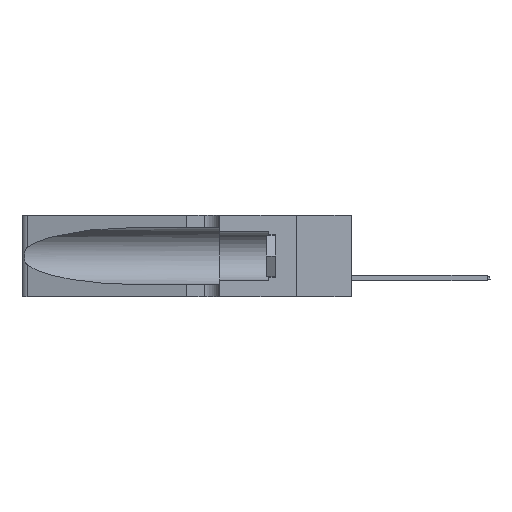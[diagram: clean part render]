
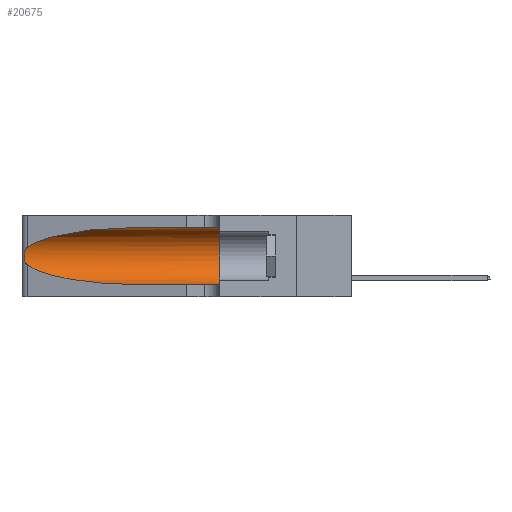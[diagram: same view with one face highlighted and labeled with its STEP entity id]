
A CAD part, left-side view. The second image highlights one B-rep face of the part: STEP entity #20675.
In plain terms, the highlighted cylindrical face has radius 3.308 mm (diameter 6.617 mm), a partial arc.
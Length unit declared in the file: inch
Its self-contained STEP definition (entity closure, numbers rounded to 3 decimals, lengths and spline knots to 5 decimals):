
#195 = ORIENTED_EDGE ( 'NONE', *, *, #631, .F. ) ;
#317 = CARTESIAN_POINT ( 'NONE',  ( 0.1305, 1.61858, 0.05475 ) ) ;
#356 = EDGE_LOOP ( 'NONE', ( #9477, #9032, #9958, #8637, #195, #3630 ) ) ;
#631 = EDGE_CURVE ( 'NONE', #19282, #6868, #21070, .T. ) ;
#970 = CARTESIAN_POINT ( 'NONE',  ( 0.25555, 1.22994, 0.2215 ) ) ;
#1056 = CARTESIAN_POINT ( 'NONE',  ( 0.25639, 1.23184, 0.21858 ) ) ;
#1067 = DIRECTION ( 'NONE',  ( 0., 1., 0. ) ) ;
#1141 = CARTESIAN_POINT ( 'NONE',  ( 0.26075, 1.23896, 0.178 ) ) ;
#1147 = AXIS2_PLACEMENT_3D ( 'NONE', #23636, #1067, #21556 ) ;
#1384 = DIRECTION ( 'NONE',  ( 0., -1., 0. ) ) ;
#1457 =( BOUNDED_CURVE ( )  B_SPLINE_CURVE ( 3, ( #15806, #17543, #21360, #10012 ),
 .UNSPECIFIED., .F., .T. ) 
 B_SPLINE_CURVE_WITH_KNOTS ( ( 4, 4 ),
 ( 3.44316, 4.71239 ),
 .UNSPECIFIED. ) 
 CURVE ( )  GEOMETRIC_REPRESENTATION_ITEM ( )  RATIONAL_B_SPLINE_CURVE ( ( 1., 0.87, 0.87, 1. ) ) 
 REPRESENTATION_ITEM ( '' )  );
#1760 = VECTOR ( 'NONE', #9818, 39.37008 ) ;
#2937 = AXIS2_PLACEMENT_3D ( 'NONE', #8709, #1384, #10711 ) ;
#2951 = CARTESIAN_POINT ( 'NONE',  ( 0.25856, 1.23593, 0.16098 ) ) ;
#3630 = ORIENTED_EDGE ( 'NONE', *, *, #8228, .F. ) ;
#4922 = VERTEX_POINT ( 'NONE', #11655 ) ;
#5606 = EDGE_CURVE ( 'NONE', #18583, #5831, #23296, .T. ) ;
#5831 = VERTEX_POINT ( 'NONE', #16990 ) ;
#6119 = VERTEX_POINT ( 'NONE', #12368 ) ;
#6274 = CARTESIAN_POINT ( 'NONE',  ( 0.18966, 0.96281, 0.31525 ) ) ;
#6665 = CARTESIAN_POINT ( 'NONE',  ( 0.26018, 1.23835, 0.19895 ) ) ;
#6868 = VERTEX_POINT ( 'NONE', #11860 ) ;
#7037 = DIRECTION ( 'NONE',  ( 0., -1., 0. ) ) ;
#7185 = CARTESIAN_POINT ( 'NONE',  ( 0.1305, 1.61858, 0.31525 ) ) ;
#7886 = FACE_OUTER_BOUND ( 'NONE', #356, .T. ) ;
#8228 = EDGE_CURVE ( 'NONE', #6119, #19282, #20398, .T. ) ;
#8541 = CARTESIAN_POINT ( 'NONE',  ( 0.26017, 1.23833, 0.17102 ) ) ;
#8637 = ORIENTED_EDGE ( 'NONE', *, *, #11089, .T. ) ;
#8709 = CARTESIAN_POINT ( 'NONE',  ( 0.1305, 1.61858, 0.185 ) ) ;
#9032 = ORIENTED_EDGE ( 'NONE', *, *, #5606, .T. ) ;
#9477 = ORIENTED_EDGE ( 'NONE', *, *, #17944, .T. ) ;
#9818 = DIRECTION ( 'NONE',  ( 0., -1., 0. ) ) ;
#9958 = ORIENTED_EDGE ( 'NONE', *, *, #12828, .T. ) ;
#10012 = CARTESIAN_POINT ( 'NONE',  ( 0.1305, 0.72297, 0.05475 ) ) ;
#10300 = CARTESIAN_POINT ( 'NONE',  ( 0.25487, 1.22718, 0.22369 ) ) ;
#10328 = VECTOR ( 'NONE', #7037, 39.37008 ) ;
#10455 = CARTESIAN_POINT ( 'NONE',  ( 0.25639, 1.23186, 0.15144 ) ) ;
#10543 = CARTESIAN_POINT ( 'NONE',  ( 0.25555, 1.22993, 0.14849 ) ) ;
#10711 = DIRECTION ( 'NONE',  ( 0., 0., -1. ) ) ;
#11089 = EDGE_CURVE ( 'NONE', #4922, #6868, #11220, .T. ) ;
#11220 = LINE ( 'NONE', #317, #1760 ) ;
#11441 = CYLINDRICAL_SURFACE ( 'NONE', #2937, 0.13025 ) ;
#11655 = CARTESIAN_POINT ( 'NONE',  ( 0.1305, 0.72297, 0.05475 ) ) ;
#11860 = CARTESIAN_POINT ( 'NONE',  ( 0.1305, 0.35, 0.05475 ) ) ;
#12368 = CARTESIAN_POINT ( 'NONE',  ( 0.1305, 0.72297, 0.31525 ) ) ;
#12828 = EDGE_CURVE ( 'NONE', #5831, #4922, #1457, .T. ) ;
#13979 = CARTESIAN_POINT ( 'NONE',  ( 0.1305, 0.72297, 0.31525 ) ) ;
#15806 = CARTESIAN_POINT ( 'NONE',  ( 0.25487, 1.22718, 0.14631 ) ) ;
#16069 = CARTESIAN_POINT ( 'NONE',  ( 0.25787, 1.23484, 0.2124 ) ) ;
#16990 = CARTESIAN_POINT ( 'NONE',  ( 0.25487, 1.22718, 0.14631 ) ) ;
#17037 = CARTESIAN_POINT ( 'NONE',  ( 0.25487, 1.22718, 0.22369 ) ) ;
#17543 = CARTESIAN_POINT ( 'NONE',  ( 0.2373, 1.15595, 0.08982 ) ) ;
#17944 = EDGE_CURVE ( 'NONE', #6119, #18583, #21134, .T. ) ;
#17983 = CARTESIAN_POINT ( 'NONE',  ( 0.25854, 1.2359, 0.20912 ) ) ;
#18057 = CARTESIAN_POINT ( 'NONE',  ( 0.25487, 1.22718, 0.14631 ) ) ;
#18583 = VERTEX_POINT ( 'NONE', #17037 ) ;
#19282 = VERTEX_POINT ( 'NONE', #19858 ) ;
#19858 = CARTESIAN_POINT ( 'NONE',  ( 0.1305, 0.35, 0.31525 ) ) ;
#19881 = CARTESIAN_POINT ( 'NONE',  ( 0.26075, 1.23896, 0.19203 ) ) ;
#20398 = LINE ( 'NONE', #7185, #10328 ) ;
#20675 = ADVANCED_FACE ( 'NONE', ( #7886 ), #11441, .F. ) ;
#21070 = CIRCLE ( 'NONE', #1147, 0.13025 ) ;
#21134 =( BOUNDED_CURVE ( )  B_SPLINE_CURVE ( 3, ( #13979, #6274, #21577, #21420 ),
 .UNSPECIFIED., .F., .T. ) 
 B_SPLINE_CURVE_WITH_KNOTS ( ( 4, 4 ),
 ( 1.5708, 2.84003 ),
 .UNSPECIFIED. ) 
 CURVE ( )  GEOMETRIC_REPRESENTATION_ITEM ( )  RATIONAL_B_SPLINE_CURVE ( ( 1., 0.87, 0.87, 1. ) ) 
 REPRESENTATION_ITEM ( '' )  );
#21360 = CARTESIAN_POINT ( 'NONE',  ( 0.18966, 0.96281, 0.05475 ) ) ;
#21420 = CARTESIAN_POINT ( 'NONE',  ( 0.25487, 1.22718, 0.22369 ) ) ;
#21556 = DIRECTION ( 'NONE',  ( 0., 0., 1. ) ) ;
#21577 = CARTESIAN_POINT ( 'NONE',  ( 0.2373, 1.15595, 0.28018 ) ) ;
#21791 = CARTESIAN_POINT ( 'NONE',  ( 0.25789, 1.23486, 0.15765 ) ) ;
#23296 = B_SPLINE_CURVE_WITH_KNOTS ( 'NONE', 3,
 ( #10300, #970, #1056, #16069, #17983, #6665, #19881, #1141, #8541, #2951, #21791, #10455, #10543, #18057 ),
 .UNSPECIFIED., .F., .F.,
 ( 4, 2, 2, 2, 2, 2, 4 ),
 ( 0., 0.00027, 0.00053, 0.00107, 0.0016, 0.00187, 0.00214 ),
 .UNSPECIFIED. ) ;
#23636 = CARTESIAN_POINT ( 'NONE',  ( 0.1305, 0.35, 0.185 ) ) ;
